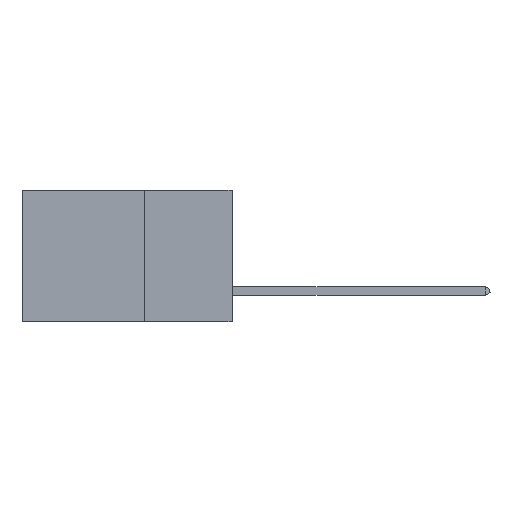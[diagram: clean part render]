
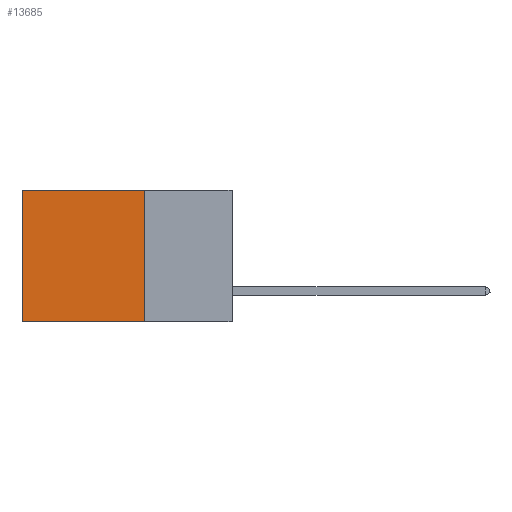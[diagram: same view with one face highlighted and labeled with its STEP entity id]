
A CAD part, left-side view. The second image highlights one B-rep face of the part: STEP entity #13685.
In plain terms, the highlighted planar face has unit normal (-1, 0, 0).
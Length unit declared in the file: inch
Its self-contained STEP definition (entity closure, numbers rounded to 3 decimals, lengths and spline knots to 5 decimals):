
#521 = CARTESIAN_POINT ( 'NONE',  ( 0.2875, 0.6, 0. ) ) ;
#789 = VECTOR ( 'NONE', #13972, 39.37008 ) ;
#961 = EDGE_CURVE ( 'NONE', #8785, #3761, #13755, .T. ) ;
#1446 = EDGE_CURVE ( 'NONE', #14197, #3761, #2144, .T. ) ;
#2032 = DIRECTION ( 'NONE',  ( 0., 0., -1. ) ) ;
#2052 = DIRECTION ( 'NONE',  ( 0., 1., 0. ) ) ;
#2144 = LINE ( 'NONE', #11561, #6238 ) ;
#2385 = CARTESIAN_POINT ( 'NONE',  ( 0.2875, 0.25, 0. ) ) ;
#3324 = DIRECTION ( 'NONE',  ( 1., 0., 0. ) ) ;
#3442 = ORIENTED_EDGE ( 'NONE', *, *, #16050, .F. ) ;
#3761 = VERTEX_POINT ( 'NONE', #13468 ) ;
#3874 = EDGE_LOOP ( 'NONE', ( #8216, #9285, #3442, #4235 ) ) ;
#4235 = ORIENTED_EDGE ( 'NONE', *, *, #11121, .T. ) ;
#4582 = CARTESIAN_POINT ( 'NONE',  ( 0.2875, 0.25, -0.375 ) ) ;
#5098 = VECTOR ( 'NONE', #2032, 39.37008 ) ;
#5186 = VERTEX_POINT ( 'NONE', #2385 ) ;
#5784 = CARTESIAN_POINT ( 'NONE',  ( 0.2875, 0.25, -0.375 ) ) ;
#6238 = VECTOR ( 'NONE', #14013, 39.37008 ) ;
#6269 = LINE ( 'NONE', #5784, #5098 ) ;
#8104 = PLANE ( 'NONE',  #12333 ) ;
#8216 = ORIENTED_EDGE ( 'NONE', *, *, #1446, .T. ) ;
#8785 = VERTEX_POINT ( 'NONE', #12991 ) ;
#9285 = ORIENTED_EDGE ( 'NONE', *, *, #961, .F. ) ;
#10192 = CARTESIAN_POINT ( 'NONE',  ( 0.2875, 0.25, -0.375 ) ) ;
#11047 = LINE ( 'NONE', #11888, #14159 ) ;
#11121 = EDGE_CURVE ( 'NONE', #5186, #14197, #11047, .T. ) ;
#11561 = CARTESIAN_POINT ( 'NONE',  ( 0.2875, 0.6, -0.375 ) ) ;
#11706 = FACE_OUTER_BOUND ( 'NONE', #3874, .T. ) ;
#11888 = CARTESIAN_POINT ( 'NONE',  ( 0.2875, 0.25, 0. ) ) ;
#11970 = DIRECTION ( 'NONE',  ( 0., 0., -1. ) ) ;
#12333 = AXIS2_PLACEMENT_3D ( 'NONE', #4582, #3324, #11970 ) ;
#12991 = CARTESIAN_POINT ( 'NONE',  ( 0.2875, 0.25, -0.375 ) ) ;
#13468 = CARTESIAN_POINT ( 'NONE',  ( 0.2875, 0.6, -0.375 ) ) ;
#13685 = ADVANCED_FACE ( 'NONE', ( #11706 ), #8104, .F. ) ;
#13755 = LINE ( 'NONE', #10192, #789 ) ;
#13972 = DIRECTION ( 'NONE',  ( 0., 1., 0. ) ) ;
#14013 = DIRECTION ( 'NONE',  ( 0., 0., -1. ) ) ;
#14159 = VECTOR ( 'NONE', #2052, 39.37008 ) ;
#14197 = VERTEX_POINT ( 'NONE', #521 ) ;
#16050 = EDGE_CURVE ( 'NONE', #5186, #8785, #6269, .T. ) ;
